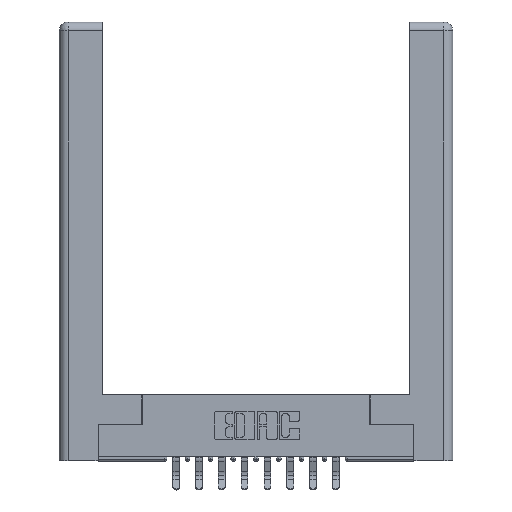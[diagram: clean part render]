
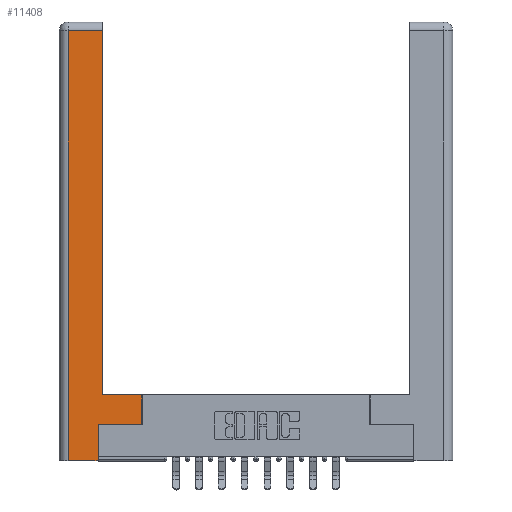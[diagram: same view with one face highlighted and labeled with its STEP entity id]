
A CAD part, top view. The second image highlights one B-rep face of the part: STEP entity #11408.
In plain terms, the highlighted planar face has unit normal (0, 0, 1).
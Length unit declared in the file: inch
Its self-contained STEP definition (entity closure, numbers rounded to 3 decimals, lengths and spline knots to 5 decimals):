
#119 = DIRECTION ( 'NONE',  ( 0., 1., 0. ) ) ;
#414 = VERTEX_POINT ( 'NONE', #8069 ) ;
#1102 = EDGE_LOOP ( 'NONE', ( #10554, #8091, #5297, #5106, #1298, #3053, #5193, #9928 ) ) ;
#1266 = VERTEX_POINT ( 'NONE', #13963 ) ;
#1298 = ORIENTED_EDGE ( 'NONE', *, *, #9158, .T. ) ;
#1604 = DIRECTION ( 'NONE',  ( 0., 0., -1. ) ) ;
#1800 = EDGE_CURVE ( 'NONE', #14465, #1266, #14291, .T. ) ;
#2076 = FACE_OUTER_BOUND ( 'NONE', #1102, .T. ) ;
#2107 = EDGE_CURVE ( 'NONE', #7428, #5880, #5395, .T. ) ;
#2311 = DIRECTION ( 'NONE',  ( 0., 1., 0. ) ) ;
#2413 = CARTESIAN_POINT ( 'NONE',  ( 0.295, 0.45, 0. ) ) ;
#2870 = EDGE_CURVE ( 'NONE', #1266, #12723, #10090, .T. ) ;
#3053 = ORIENTED_EDGE ( 'NONE', *, *, #2107, .T. ) ;
#3237 = CARTESIAN_POINT ( 'NONE',  ( 0.295, 0.45, 0. ) ) ;
#3593 = EDGE_CURVE ( 'NONE', #10080, #14715, #7800, .T. ) ;
#3911 = EDGE_CURVE ( 'NONE', #12723, #10080, #12127, .T. ) ;
#4022 = VECTOR ( 'NONE', #4549, 39.37008 ) ;
#4066 = LINE ( 'NONE', #2413, #6523 ) ;
#4549 = DIRECTION ( 'NONE',  ( 0., -1., 0. ) ) ;
#4991 = CARTESIAN_POINT ( 'NONE',  ( 0.265, 0., 0. ) ) ;
#5106 = ORIENTED_EDGE ( 'NONE', *, *, #3593, .T. ) ;
#5193 = ORIENTED_EDGE ( 'NONE', *, *, #5567, .T. ) ;
#5297 = ORIENTED_EDGE ( 'NONE', *, *, #3911, .T. ) ;
#5395 = LINE ( 'NONE', #13171, #10294 ) ;
#5567 = EDGE_CURVE ( 'NONE', #5880, #414, #14642, .T. ) ;
#5605 = CARTESIAN_POINT ( 'NONE',  ( 0.0615, 2.94, 0. ) ) ;
#5880 = VERTEX_POINT ( 'NONE', #11341 ) ;
#5931 = EDGE_CURVE ( 'NONE', #414, #14465, #4066, .T. ) ;
#5938 = DIRECTION ( 'NONE',  ( 1., 0., 0. ) ) ;
#6006 = CARTESIAN_POINT ( 'NONE',  ( 0.265, 0.245, 0. ) ) ;
#6032 = CARTESIAN_POINT ( 'NONE',  ( 0.565, 0.45, 0. ) ) ;
#6112 = DIRECTION ( 'NONE',  ( -1., 0., 0. ) ) ;
#6124 = DIRECTION ( 'NONE',  ( 0., 1., 0. ) ) ;
#6523 = VECTOR ( 'NONE', #6112, 39.37008 ) ;
#6712 = VECTOR ( 'NONE', #119, 39.37008 ) ;
#7159 = CARTESIAN_POINT ( 'NONE',  ( 0.265, 0., 0. ) ) ;
#7172 = LINE ( 'NONE', #9591, #7551 ) ;
#7428 = VERTEX_POINT ( 'NONE', #6006 ) ;
#7551 = VECTOR ( 'NONE', #2311, 39.37008 ) ;
#7800 = LINE ( 'NONE', #7159, #13858 ) ;
#8069 = CARTESIAN_POINT ( 'NONE',  ( 0.565, 0.45, 0. ) ) ;
#8091 = ORIENTED_EDGE ( 'NONE', *, *, #2870, .T. ) ;
#8199 = DIRECTION ( 'NONE',  ( 1., 0., 0. ) ) ;
#8240 = CARTESIAN_POINT ( 'NONE',  ( 0.0615, 0., 0. ) ) ;
#8497 = CARTESIAN_POINT ( 'NONE',  ( 0.0615, 2.94, 0. ) ) ;
#8868 = CARTESIAN_POINT ( 'NONE',  ( 0., 0., 0. ) ) ;
#9158 = EDGE_CURVE ( 'NONE', #14715, #7428, #7172, .T. ) ;
#9591 = CARTESIAN_POINT ( 'NONE',  ( 0.265, 0.245, 0. ) ) ;
#9928 = ORIENTED_EDGE ( 'NONE', *, *, #5931, .T. ) ;
#10080 = VERTEX_POINT ( 'NONE', #13159 ) ;
#10090 = LINE ( 'NONE', #8497, #11241 ) ;
#10231 = PLANE ( 'NONE',  #10705 ) ;
#10294 = VECTOR ( 'NONE', #5938, 39.37008 ) ;
#10554 = ORIENTED_EDGE ( 'NONE', *, *, #1800, .T. ) ;
#10705 = AXIS2_PLACEMENT_3D ( 'NONE', #8868, #1604, #13736 ) ;
#10917 = CARTESIAN_POINT ( 'NONE',  ( 0.295, 3., 0. ) ) ;
#11241 = VECTOR ( 'NONE', #13628, 39.37008 ) ;
#11341 = CARTESIAN_POINT ( 'NONE',  ( 0.565, 0.245, 0. ) ) ;
#11408 = ADVANCED_FACE ( 'NONE', ( #2076 ), #10231, .F. ) ;
#12127 = LINE ( 'NONE', #8240, #4022 ) ;
#12723 = VERTEX_POINT ( 'NONE', #5605 ) ;
#13159 = CARTESIAN_POINT ( 'NONE',  ( 0.0615, 0., 0. ) ) ;
#13171 = CARTESIAN_POINT ( 'NONE',  ( 0.565, 0.245, 0. ) ) ;
#13551 = VECTOR ( 'NONE', #6124, 39.37008 ) ;
#13628 = DIRECTION ( 'NONE',  ( -1., 0., 0. ) ) ;
#13736 = DIRECTION ( 'NONE',  ( -1., 0., 0. ) ) ;
#13858 = VECTOR ( 'NONE', #8199, 39.37008 ) ;
#13963 = CARTESIAN_POINT ( 'NONE',  ( 0.295, 2.94, 0. ) ) ;
#14291 = LINE ( 'NONE', #10917, #13551 ) ;
#14465 = VERTEX_POINT ( 'NONE', #3237 ) ;
#14642 = LINE ( 'NONE', #6032, #6712 ) ;
#14715 = VERTEX_POINT ( 'NONE', #4991 ) ;
